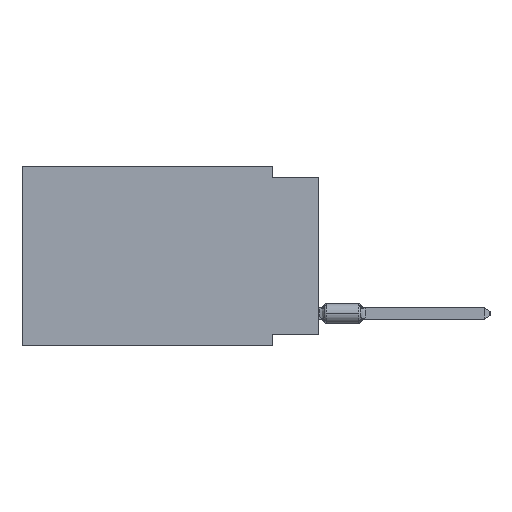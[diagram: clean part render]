
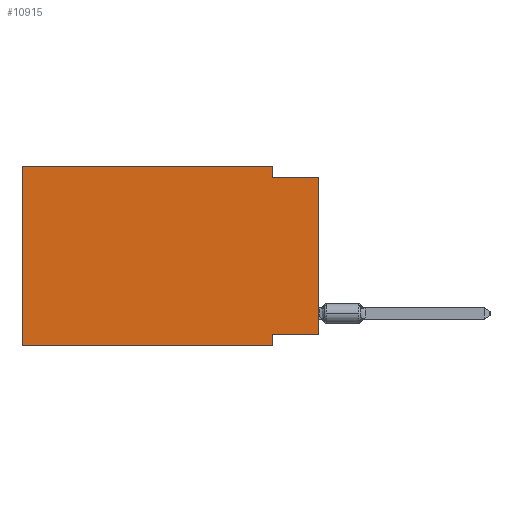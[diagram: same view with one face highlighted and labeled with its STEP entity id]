
A CAD part, left-side view. The second image highlights one B-rep face of the part: STEP entity #10915.
In plain terms, the highlighted planar face has unit normal (-1, 0, 0).
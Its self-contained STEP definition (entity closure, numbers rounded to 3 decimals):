
#400 = ORIENTED_EDGE ( 'NONE', *, *, #33214, .F. ) ;
#547 = VERTEX_POINT ( 'NONE', #51342 ) ;
#2371 = VERTEX_POINT ( 'NONE', #2656 ) ;
#2656 = CARTESIAN_POINT ( 'NONE',  ( 0., 16.383, -9.906 ) ) ;
#3575 = CARTESIAN_POINT ( 'NONE',  ( 0., 16.383, 0. ) ) ;
#5097 = ORIENTED_EDGE ( 'NONE', *, *, #12931, .T. ) ;
#5345 = DIRECTION ( 'NONE',  ( 0., -1., 0. ) ) ;
#6930 = ORIENTED_EDGE ( 'NONE', *, *, #33511, .F. ) ;
#7321 = VERTEX_POINT ( 'NONE', #3575 ) ;
#7503 = VECTOR ( 'NONE', #48977, 1000. ) ;
#7929 = VERTEX_POINT ( 'NONE', #22026 ) ;
#8758 = VECTOR ( 'NONE', #16912, 1000. ) ;
#8856 = LINE ( 'NONE', #48679, #24748 ) ;
#10392 = LINE ( 'NONE', #51496, #51006 ) ;
#10915 = ADVANCED_FACE ( 'NONE', ( #11015 ), #28295, .F. ) ;
#10964 = EDGE_LOOP ( 'NONE', ( #5097, #31873, #23129, #15870, #400, #42817, #6930, #20521 ) ) ;
#11015 = FACE_OUTER_BOUND ( 'NONE', #10964, .T. ) ;
#11218 = CARTESIAN_POINT ( 'NONE',  ( 0., 0., -0.635 ) ) ;
#11566 = CARTESIAN_POINT ( 'NONE',  ( 0., 2.54, 0. ) ) ;
#11929 = CARTESIAN_POINT ( 'NONE',  ( 0., 16.383, -9.906 ) ) ;
#12056 = VECTOR ( 'NONE', #16455, 1000. ) ;
#12931 = EDGE_CURVE ( 'NONE', #547, #33622, #10392, .T. ) ;
#13065 = EDGE_CURVE ( 'NONE', #2371, #33249, #16188, .T. ) ;
#14570 = EDGE_CURVE ( 'NONE', #7929, #33622, #35659, .T. ) ;
#15140 = AXIS2_PLACEMENT_3D ( 'NONE', #44460, #24055, #51363 ) ;
#15522 = VECTOR ( 'NONE', #5345, 1000. ) ;
#15870 = ORIENTED_EDGE ( 'NONE', *, *, #32460, .F. ) ;
#16188 = LINE ( 'NONE', #11929, #12056 ) ;
#16455 = DIRECTION ( 'NONE',  ( 0., -1., 0. ) ) ;
#16912 = DIRECTION ( 'NONE',  ( 0., 0., 1. ) ) ;
#18348 = DIRECTION ( 'NONE',  ( 0., 0., 1. ) ) ;
#20521 = ORIENTED_EDGE ( 'NONE', *, *, #30717, .F. ) ;
#22026 = CARTESIAN_POINT ( 'NONE',  ( 0., 2.54, -0.635 ) ) ;
#23111 = VECTOR ( 'NONE', #37551, 1000. ) ;
#23129 = ORIENTED_EDGE ( 'NONE', *, *, #29104, .F. ) ;
#24055 = DIRECTION ( 'NONE',  ( 1., 0., 0. ) ) ;
#24193 = CARTESIAN_POINT ( 'NONE',  ( 0., 0., -0.635 ) ) ;
#24748 = VECTOR ( 'NONE', #40206, 1000. ) ;
#27444 = DIRECTION ( 'NONE',  ( 0., -1., 0. ) ) ;
#28295 = PLANE ( 'NONE',  #15140 ) ;
#29104 = EDGE_CURVE ( 'NONE', #51859, #7929, #40774, .T. ) ;
#29942 = CARTESIAN_POINT ( 'NONE',  ( 0., 16.383, 0. ) ) ;
#30717 = EDGE_CURVE ( 'NONE', #547, #49590, #8856, .T. ) ;
#31873 = ORIENTED_EDGE ( 'NONE', *, *, #14570, .F. ) ;
#32460 = EDGE_CURVE ( 'NONE', #7321, #51859, #34305, .T. ) ;
#33214 = EDGE_CURVE ( 'NONE', #2371, #7321, #33908, .T. ) ;
#33249 = VERTEX_POINT ( 'NONE', #45047 ) ;
#33308 = CARTESIAN_POINT ( 'NONE',  ( 0., 2.54, -9.906 ) ) ;
#33352 = CARTESIAN_POINT ( 'NONE',  ( 0., 2.54, 0. ) ) ;
#33511 = EDGE_CURVE ( 'NONE', #49590, #33249, #41798, .T. ) ;
#33622 = VERTEX_POINT ( 'NONE', #24193 ) ;
#33908 = LINE ( 'NONE', #29942, #8758 ) ;
#34305 = LINE ( 'NONE', #50198, #15522 ) ;
#35659 = LINE ( 'NONE', #11218, #45404 ) ;
#37551 = DIRECTION ( 'NONE',  ( 0., 0., -1. ) ) ;
#40206 = DIRECTION ( 'NONE',  ( 0., 1., 0. ) ) ;
#40774 = LINE ( 'NONE', #11566, #7503 ) ;
#41798 = LINE ( 'NONE', #33308, #23111 ) ;
#42817 = ORIENTED_EDGE ( 'NONE', *, *, #13065, .T. ) ;
#44460 = CARTESIAN_POINT ( 'NONE',  ( 0., 16.383, 0. ) ) ;
#45047 = CARTESIAN_POINT ( 'NONE',  ( 0., 2.54, -9.906 ) ) ;
#45404 = VECTOR ( 'NONE', #27444, 1000. ) ;
#47012 = CARTESIAN_POINT ( 'NONE',  ( 0., 2.54, -9.271 ) ) ;
#48679 = CARTESIAN_POINT ( 'NONE',  ( 0., 0., -9.271 ) ) ;
#48977 = DIRECTION ( 'NONE',  ( 0., 0., -1. ) ) ;
#49590 = VERTEX_POINT ( 'NONE', #47012 ) ;
#50198 = CARTESIAN_POINT ( 'NONE',  ( 0., 16.383, 0. ) ) ;
#51006 = VECTOR ( 'NONE', #18348, 1000. ) ;
#51342 = CARTESIAN_POINT ( 'NONE',  ( 0., 0., -9.271 ) ) ;
#51363 = DIRECTION ( 'NONE',  ( 0., 0., -1. ) ) ;
#51496 = CARTESIAN_POINT ( 'NONE',  ( 0., 0., 0. ) ) ;
#51859 = VERTEX_POINT ( 'NONE', #33352 ) ;
